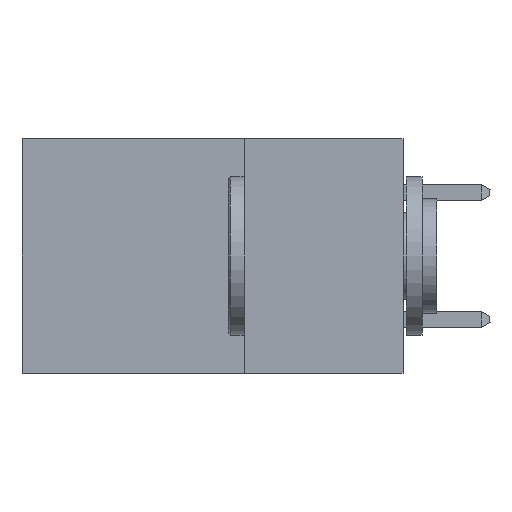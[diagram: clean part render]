
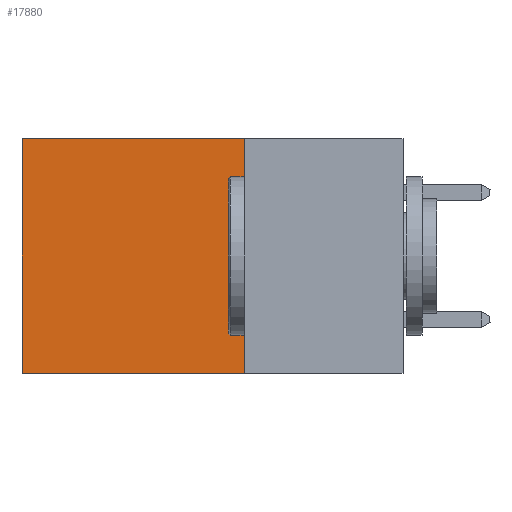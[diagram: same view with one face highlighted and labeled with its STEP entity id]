
A CAD part, left-side view. The second image highlights one B-rep face of the part: STEP entity #17880.
In plain terms, the highlighted planar face has unit normal (-1, 0, 0).
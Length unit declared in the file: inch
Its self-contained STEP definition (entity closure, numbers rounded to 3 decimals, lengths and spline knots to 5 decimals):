
#52 = ORIENTED_EDGE ( 'NONE', *, *, #7250, .F. ) ;
#1551 = VERTEX_POINT ( 'NONE', #13001 ) ;
#2029 = ORIENTED_EDGE ( 'NONE', *, *, #13554, .T. ) ;
#3948 = VECTOR ( 'NONE', #22831, 39.37008 ) ;
#4650 = EDGE_CURVE ( 'NONE', #4747, #1551, #18282, .T. ) ;
#4747 = VERTEX_POINT ( 'NONE', #19563 ) ;
#5616 = AXIS2_PLACEMENT_3D ( 'NONE', #22691, #19194, #8494 ) ;
#5753 = CARTESIAN_POINT ( 'NONE',  ( 0.2875, 0.25, -0.37 ) ) ;
#5949 = LINE ( 'NONE', #19450, #16059 ) ;
#6681 = PLANE ( 'NONE',  #5616 ) ;
#6735 = VECTOR ( 'NONE', #15372, 39.37008 ) ;
#7250 = EDGE_CURVE ( 'NONE', #1551, #14544, #10622, .T. ) ;
#8494 = DIRECTION ( 'NONE',  ( 0., 0., -1. ) ) ;
#8753 = DIRECTION ( 'NONE',  ( 0., 1., 0. ) ) ;
#10622 = LINE ( 'NONE', #5753, #19559 ) ;
#11502 = LINE ( 'NONE', #20733, #6735 ) ;
#12721 = VERTEX_POINT ( 'NONE', #18675 ) ;
#12851 = FACE_OUTER_BOUND ( 'NONE', #18553, .T. ) ;
#13001 = CARTESIAN_POINT ( 'NONE',  ( 0.2875, 0.25, -0.37 ) ) ;
#13554 = EDGE_CURVE ( 'NONE', #12721, #14544, #11502, .T. ) ;
#14544 = VERTEX_POINT ( 'NONE', #20074 ) ;
#15372 = DIRECTION ( 'NONE',  ( 0., 0., -1. ) ) ;
#15570 = ORIENTED_EDGE ( 'NONE', *, *, #4650, .F. ) ;
#16059 = VECTOR ( 'NONE', #8753, 39.37008 ) ;
#17572 = CARTESIAN_POINT ( 'NONE',  ( 0.2875, 0.25, 0. ) ) ;
#17880 = ADVANCED_FACE ( 'NONE', ( #12851 ), #6681, .F. ) ;
#18282 = LINE ( 'NONE', #17572, #3948 ) ;
#18553 = EDGE_LOOP ( 'NONE', ( #2029, #52, #15570, #22341 ) ) ;
#18675 = CARTESIAN_POINT ( 'NONE',  ( 0.2875, 0.6, 0. ) ) ;
#19194 = DIRECTION ( 'NONE',  ( 1., 0., 0. ) ) ;
#19450 = CARTESIAN_POINT ( 'NONE',  ( 0.2875, 0.25, 0. ) ) ;
#19559 = VECTOR ( 'NONE', #21872, 39.37008 ) ;
#19563 = CARTESIAN_POINT ( 'NONE',  ( 0.2875, 0.25, 0. ) ) ;
#20074 = CARTESIAN_POINT ( 'NONE',  ( 0.2875, 0.6, -0.37 ) ) ;
#20733 = CARTESIAN_POINT ( 'NONE',  ( 0.2875, 0.6, 0. ) ) ;
#21872 = DIRECTION ( 'NONE',  ( 0., 1., 0. ) ) ;
#22341 = ORIENTED_EDGE ( 'NONE', *, *, #22982, .T. ) ;
#22691 = CARTESIAN_POINT ( 'NONE',  ( 0.2875, 0.25, 0. ) ) ;
#22831 = DIRECTION ( 'NONE',  ( 0., 0., -1. ) ) ;
#22982 = EDGE_CURVE ( 'NONE', #4747, #12721, #5949, .T. ) ;
